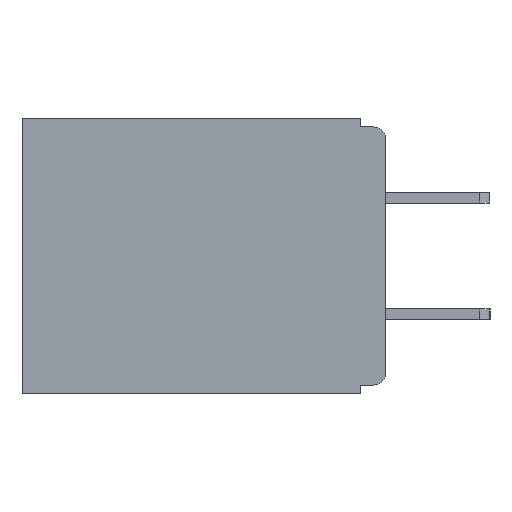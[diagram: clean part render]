
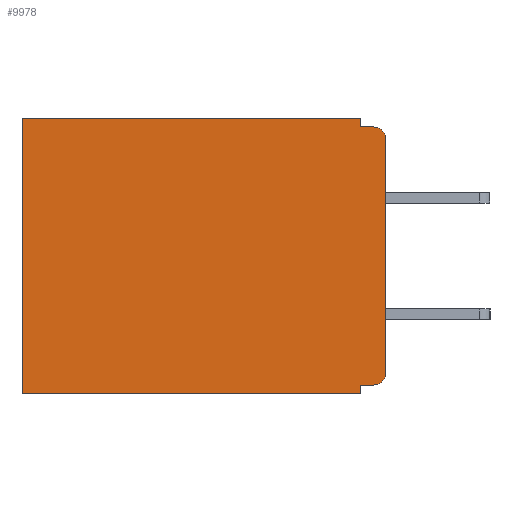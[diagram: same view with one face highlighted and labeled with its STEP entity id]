
A CAD part, left-side view. The second image highlights one B-rep face of the part: STEP entity #9978.
In plain terms, the highlighted planar face has unit normal (-1, 0, 0).
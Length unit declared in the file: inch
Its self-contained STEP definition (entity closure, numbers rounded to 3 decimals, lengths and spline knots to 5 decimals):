
#296 = VERTEX_POINT ( 'NONE', #8688 ) ;
#612 = VERTEX_POINT ( 'NONE', #17009 ) ;
#672 = ORIENTED_EDGE ( 'NONE', *, *, #13950, .F. ) ;
#789 = LINE ( 'NONE', #3053, #15005 ) ;
#945 = CIRCLE ( 'NONE', #3228, 0.015 ) ;
#1446 = VERTEX_POINT ( 'NONE', #16369 ) ;
#1708 = CARTESIAN_POINT ( 'NONE',  ( 0.3, 0.015, -0.305 ) ) ;
#1754 = CARTESIAN_POINT ( 'NONE',  ( 0.3, 0., -0.33 ) ) ;
#1956 = DIRECTION ( 'NONE',  ( 0., 1., 0. ) ) ;
#1989 = LINE ( 'NONE', #13940, #8704 ) ;
#2252 = CARTESIAN_POINT ( 'NONE',  ( 0.3, 0., -0.33 ) ) ;
#2266 = EDGE_CURVE ( 'NONE', #4794, #612, #15275, .T. ) ;
#3053 = CARTESIAN_POINT ( 'NONE',  ( 0.3, 0.031, 0. ) ) ;
#3090 = DIRECTION ( 'NONE',  ( 0., 0., -1. ) ) ;
#3203 = CARTESIAN_POINT ( 'NONE',  ( 0.3, 0.015, -0.32 ) ) ;
#3228 = AXIS2_PLACEMENT_3D ( 'NONE', #8791, #8775, #8757 ) ;
#3240 = VERTEX_POINT ( 'NONE', #8295 ) ;
#3701 = DIRECTION ( 'NONE',  ( 0., 0., -1. ) ) ;
#3739 = DIRECTION ( 'NONE',  ( 1., 0., 0. ) ) ;
#3896 = EDGE_LOOP ( 'NONE', ( #6079, #14015, #672, #12760, #11613, #13623, #13882, #5079, #11977, #16995 ) ) ;
#4193 = DIRECTION ( 'NONE',  ( 0., 0., -1. ) ) ;
#4209 = CARTESIAN_POINT ( 'NONE',  ( 0.3, 0.031, -0.33 ) ) ;
#4241 = DIRECTION ( 'NONE',  ( 0., 0., -1. ) ) ;
#4321 = EDGE_CURVE ( 'NONE', #13342, #612, #5013, .T. ) ;
#4586 = VERTEX_POINT ( 'NONE', #9115 ) ;
#4777 = CARTESIAN_POINT ( 'NONE',  ( 0.3, 0.015, -0.01 ) ) ;
#4794 = VERTEX_POINT ( 'NONE', #15621 ) ;
#4937 = PLANE ( 'NONE',  #11399 ) ;
#5013 = CIRCLE ( 'NONE', #10528, 0.015 ) ;
#5079 = ORIENTED_EDGE ( 'NONE', *, *, #13251, .F. ) ;
#5122 = LINE ( 'NONE', #6494, #11428 ) ;
#6079 = ORIENTED_EDGE ( 'NONE', *, *, #2266, .F. ) ;
#6494 = CARTESIAN_POINT ( 'NONE',  ( 0.3, 0.437, -0.33 ) ) ;
#6658 = EDGE_CURVE ( 'NONE', #296, #1446, #1989, .T. ) ;
#6702 = DIRECTION ( 'NONE',  ( 0., -1., 0. ) ) ;
#6735 = CARTESIAN_POINT ( 'NONE',  ( 0.3, 0., -0.33 ) ) ;
#7182 = VECTOR ( 'NONE', #4193, 39.37008 ) ;
#7227 = VERTEX_POINT ( 'NONE', #11897 ) ;
#7648 = EDGE_CURVE ( 'NONE', #4586, #11884, #7849, .T. ) ;
#7849 = LINE ( 'NONE', #6735, #12263 ) ;
#8295 = CARTESIAN_POINT ( 'NONE',  ( 0.3, 0.031, -0.01 ) ) ;
#8688 = CARTESIAN_POINT ( 'NONE',  ( 0.3, 0.031, 0. ) ) ;
#8704 = VECTOR ( 'NONE', #13646, 39.37008 ) ;
#8757 = DIRECTION ( 'NONE',  ( 0., 0., -1. ) ) ;
#8775 = DIRECTION ( 'NONE',  ( -1., 0., 0. ) ) ;
#8791 = CARTESIAN_POINT ( 'NONE',  ( 0.3, 0.015, -0.025 ) ) ;
#8819 = LINE ( 'NONE', #11222, #16978 ) ;
#9112 = EDGE_CURVE ( 'NONE', #13342, #7227, #8819, .T. ) ;
#9115 = CARTESIAN_POINT ( 'NONE',  ( 0.3, 0.031, -0.33 ) ) ;
#9171 = DIRECTION ( 'NONE',  ( 0., 0., -1. ) ) ;
#9626 = FACE_OUTER_BOUND ( 'NONE', #3896, .T. ) ;
#9847 = DIRECTION ( 'NONE',  ( -1., 0., 0. ) ) ;
#9978 = ADVANCED_FACE ( 'NONE', ( #9626 ), #4937, .F. ) ;
#10226 = DIRECTION ( 'NONE',  ( 0., 1., 0. ) ) ;
#10528 = AXIS2_PLACEMENT_3D ( 'NONE', #1708, #9847, #4241 ) ;
#10550 = EDGE_CURVE ( 'NONE', #296, #3240, #789, .T. ) ;
#11222 = CARTESIAN_POINT ( 'NONE',  ( 0.3, 0., -0.32 ) ) ;
#11399 = AXIS2_PLACEMENT_3D ( 'NONE', #1754, #3739, #3701 ) ;
#11428 = VECTOR ( 'NONE', #9171, 39.37008 ) ;
#11613 = ORIENTED_EDGE ( 'NONE', *, *, #6658, .T. ) ;
#11884 = VERTEX_POINT ( 'NONE', #15832 ) ;
#11897 = CARTESIAN_POINT ( 'NONE',  ( 0.3, 0.031, -0.32 ) ) ;
#11977 = ORIENTED_EDGE ( 'NONE', *, *, #9112, .F. ) ;
#12263 = VECTOR ( 'NONE', #1956, 39.37008 ) ;
#12745 = EDGE_CURVE ( 'NONE', #4794, #15421, #945, .T. ) ;
#12760 = ORIENTED_EDGE ( 'NONE', *, *, #10550, .F. ) ;
#12796 = VECTOR ( 'NONE', #6702, 39.37008 ) ;
#13217 = LINE ( 'NONE', #13379, #12796 ) ;
#13251 = EDGE_CURVE ( 'NONE', #7227, #4586, #13853, .T. ) ;
#13342 = VERTEX_POINT ( 'NONE', #3203 ) ;
#13379 = CARTESIAN_POINT ( 'NONE',  ( 0.3, 0., -0.01 ) ) ;
#13623 = ORIENTED_EDGE ( 'NONE', *, *, #17034, .T. ) ;
#13646 = DIRECTION ( 'NONE',  ( 0., 1., 0. ) ) ;
#13853 = LINE ( 'NONE', #4209, #7182 ) ;
#13882 = ORIENTED_EDGE ( 'NONE', *, *, #7648, .F. ) ;
#13940 = CARTESIAN_POINT ( 'NONE',  ( 0.3, 0., 0. ) ) ;
#13950 = EDGE_CURVE ( 'NONE', #3240, #15421, #13217, .T. ) ;
#14015 = ORIENTED_EDGE ( 'NONE', *, *, #12745, .T. ) ;
#14899 = VECTOR ( 'NONE', #15410, 39.37008 ) ;
#15005 = VECTOR ( 'NONE', #3090, 39.37008 ) ;
#15275 = LINE ( 'NONE', #2252, #14899 ) ;
#15410 = DIRECTION ( 'NONE',  ( 0., 0., -1. ) ) ;
#15421 = VERTEX_POINT ( 'NONE', #4777 ) ;
#15621 = CARTESIAN_POINT ( 'NONE',  ( 0.3, 0., -0.025 ) ) ;
#15832 = CARTESIAN_POINT ( 'NONE',  ( 0.3, 0.437, -0.33 ) ) ;
#16369 = CARTESIAN_POINT ( 'NONE',  ( 0.3, 0.437, 0. ) ) ;
#16978 = VECTOR ( 'NONE', #10226, 39.37008 ) ;
#16995 = ORIENTED_EDGE ( 'NONE', *, *, #4321, .T. ) ;
#17009 = CARTESIAN_POINT ( 'NONE',  ( 0.3, 0., -0.305 ) ) ;
#17034 = EDGE_CURVE ( 'NONE', #1446, #11884, #5122, .T. ) ;
